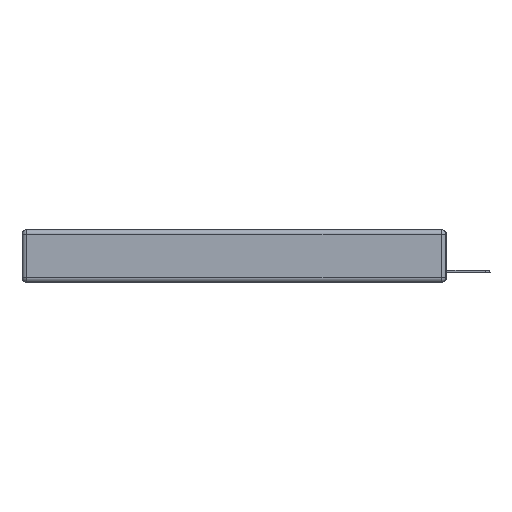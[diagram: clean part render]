
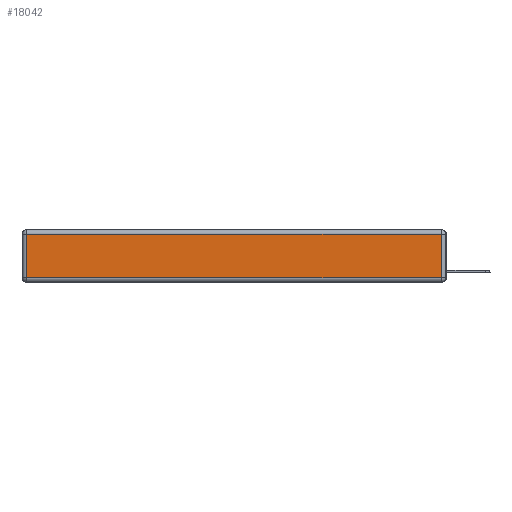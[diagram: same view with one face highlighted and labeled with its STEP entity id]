
A CAD part, left-side view. The second image highlights one B-rep face of the part: STEP entity #18042.
In plain terms, the highlighted planar face has unit normal (-1, 0, 0).
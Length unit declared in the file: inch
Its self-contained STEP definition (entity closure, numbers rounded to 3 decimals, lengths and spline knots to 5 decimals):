
#1073 = ORIENTED_EDGE ( 'NONE', *, *, #18206, .T. ) ;
#1428 = VERTEX_POINT ( 'NONE', #4590 ) ;
#1739 = DIRECTION ( 'NONE',  ( 0., 0., 1. ) ) ;
#2449 = EDGE_LOOP ( 'NONE', ( #1073, #14303, #14746, #3035 ) ) ;
#2656 = EDGE_CURVE ( 'NONE', #7714, #9843, #19939, .T. ) ;
#3035 = ORIENTED_EDGE ( 'NONE', *, *, #19522, .T. ) ;
#3484 = CARTESIAN_POINT ( 'NONE',  ( 0., 2.75, -0.03 ) ) ;
#3603 = DIRECTION ( 'NONE',  ( 0., 0., 1. ) ) ;
#4590 = CARTESIAN_POINT ( 'NONE',  ( 0., 2.72, -0.313 ) ) ;
#4746 = CARTESIAN_POINT ( 'NONE',  ( 0., 2.72, -0.03 ) ) ;
#4794 = LINE ( 'NONE', #10780, #12138 ) ;
#6078 = LINE ( 'NONE', #3484, #10942 ) ;
#7714 = VERTEX_POINT ( 'NONE', #13709 ) ;
#9548 = VERTEX_POINT ( 'NONE', #4746 ) ;
#9843 = VERTEX_POINT ( 'NONE', #10000 ) ;
#10000 = CARTESIAN_POINT ( 'NONE',  ( 0., 0.03, -0.03 ) ) ;
#10502 = AXIS2_PLACEMENT_3D ( 'NONE', #17760, #16093, #3603 ) ;
#10537 = VECTOR ( 'NONE', #1739, 39.37008 ) ;
#10780 = CARTESIAN_POINT ( 'NONE',  ( 0., 2.72, -0.343 ) ) ;
#10942 = VECTOR ( 'NONE', #16178, 39.37008 ) ;
#11276 = PLANE ( 'NONE',  #10502 ) ;
#11455 = VECTOR ( 'NONE', #20151, 39.37008 ) ;
#12138 = VECTOR ( 'NONE', #15260, 39.37008 ) ;
#13681 = LINE ( 'NONE', #18735, #11455 ) ;
#13709 = CARTESIAN_POINT ( 'NONE',  ( 0., 0.03, -0.313 ) ) ;
#14303 = ORIENTED_EDGE ( 'NONE', *, *, #2656, .T. ) ;
#14746 = ORIENTED_EDGE ( 'NONE', *, *, #18496, .T. ) ;
#15260 = DIRECTION ( 'NONE',  ( 0., 0., -1. ) ) ;
#16093 = DIRECTION ( 'NONE',  ( -1., 0., 0. ) ) ;
#16178 = DIRECTION ( 'NONE',  ( 0., 1., 0. ) ) ;
#17760 = CARTESIAN_POINT ( 'NONE',  ( 0., 0., -0.343 ) ) ;
#18042 = ADVANCED_FACE ( 'NONE', ( #19357 ), #11276, .T. ) ;
#18206 = EDGE_CURVE ( 'NONE', #1428, #7714, #13681, .T. ) ;
#18496 = EDGE_CURVE ( 'NONE', #9843, #9548, #6078, .T. ) ;
#18735 = CARTESIAN_POINT ( 'NONE',  ( 0., 0., -0.313 ) ) ;
#18994 = CARTESIAN_POINT ( 'NONE',  ( 0., 0.03, -0.343 ) ) ;
#19357 = FACE_OUTER_BOUND ( 'NONE', #2449, .T. ) ;
#19522 = EDGE_CURVE ( 'NONE', #9548, #1428, #4794, .T. ) ;
#19939 = LINE ( 'NONE', #18994, #10537 ) ;
#20151 = DIRECTION ( 'NONE',  ( 0., -1., 0. ) ) ;
